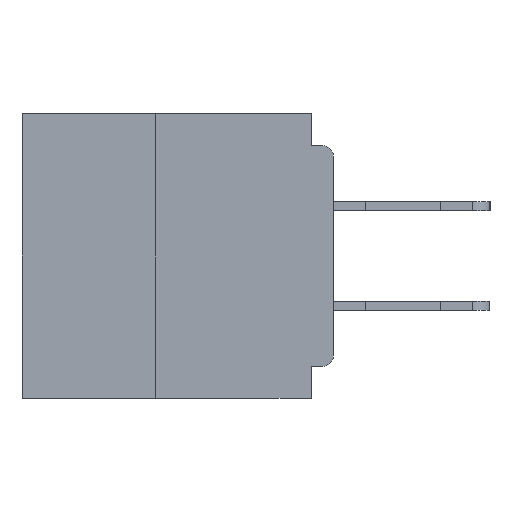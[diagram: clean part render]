
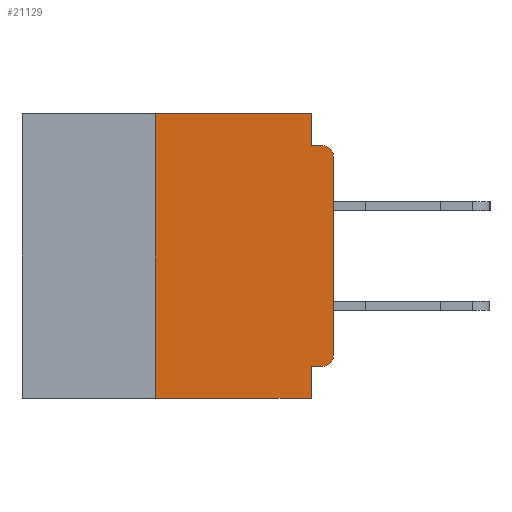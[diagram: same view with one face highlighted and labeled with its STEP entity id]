
A CAD part, left-side view. The second image highlights one B-rep face of the part: STEP entity #21129.
In plain terms, the highlighted planar face has unit normal (-1, 0, 0).
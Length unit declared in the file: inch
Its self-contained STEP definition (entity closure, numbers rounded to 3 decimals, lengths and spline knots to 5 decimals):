
#34 = FACE_OUTER_BOUND ( 'NONE', #45050, .T. ) ;
#398 = CARTESIAN_POINT ( 'NONE',  ( 0., 0.437, -0.4 ) ) ;
#819 = VERTEX_POINT ( 'NONE', #7187 ) ;
#1262 = ORIENTED_EDGE ( 'NONE', *, *, #8777, .F. ) ;
#2060 = LINE ( 'NONE', #12299, #20236 ) ;
#2630 = CARTESIAN_POINT ( 'NONE',  ( 0., 0., 0. ) ) ;
#4308 = VECTOR ( 'NONE', #33841, 39.37008 ) ;
#4326 = LINE ( 'NONE', #37947, #33283 ) ;
#5085 = CARTESIAN_POINT ( 'NONE',  ( 0., 0.031, -0.355 ) ) ;
#5507 = AXIS2_PLACEMENT_3D ( 'NONE', #33290, #11552, #36946 ) ;
#7187 = CARTESIAN_POINT ( 'NONE',  ( 0., 0., -0.34 ) ) ;
#7574 = VERTEX_POINT ( 'NONE', #23682 ) ;
#7761 = DIRECTION ( 'NONE',  ( 0., -1., 0. ) ) ;
#7824 = CARTESIAN_POINT ( 'NONE',  ( 0., 0., -0.045 ) ) ;
#8777 = EDGE_CURVE ( 'NONE', #12521, #19618, #2060, .T. ) ;
#9501 = CARTESIAN_POINT ( 'NONE',  ( 0., 0.437, 0. ) ) ;
#10385 = EDGE_CURVE ( 'NONE', #12523, #819, #18390, .T. ) ;
#10582 = CARTESIAN_POINT ( 'NONE',  ( 0., 0.25, -0.4 ) ) ;
#10930 = CARTESIAN_POINT ( 'NONE',  ( 0., 0., -0.355 ) ) ;
#11438 = DIRECTION ( 'NONE',  ( 0., -1., 0. ) ) ;
#11552 = DIRECTION ( 'NONE',  ( -1., 0., 0. ) ) ;
#11777 = CIRCLE ( 'NONE', #5507, 0.015 ) ;
#12271 = VECTOR ( 'NONE', #7761, 39.37008 ) ;
#12299 = CARTESIAN_POINT ( 'NONE',  ( 0., 0.031, -0.4 ) ) ;
#12521 = VERTEX_POINT ( 'NONE', #5085 ) ;
#12523 = VERTEX_POINT ( 'NONE', #37447 ) ;
#12572 = DIRECTION ( 'NONE',  ( 0., 0., 1. ) ) ;
#13108 = DIRECTION ( 'NONE',  ( 1., 0., 0. ) ) ;
#13409 = ORIENTED_EDGE ( 'NONE', *, *, #14032, .T. ) ;
#13420 = DIRECTION ( 'NONE',  ( 0., 0., 1. ) ) ;
#13845 = VECTOR ( 'NONE', #13420, 39.37008 ) ;
#14032 = EDGE_CURVE ( 'NONE', #819, #38822, #42733, .T. ) ;
#15347 = DIRECTION ( 'NONE',  ( 0., -1., 0. ) ) ;
#15557 = VECTOR ( 'NONE', #32649, 39.37008 ) ;
#15953 = DIRECTION ( 'NONE',  ( 0., 0., -1. ) ) ;
#17094 = VERTEX_POINT ( 'NONE', #43272 ) ;
#17289 = ORIENTED_EDGE ( 'NONE', *, *, #41029, .F. ) ;
#17825 = LINE ( 'NONE', #10930, #15557 ) ;
#18379 = CARTESIAN_POINT ( 'NONE',  ( 0., 0.015, -0.34 ) ) ;
#18390 = CIRCLE ( 'NONE', #34389, 0.015 ) ;
#18498 = EDGE_CURVE ( 'NONE', #33064, #19618, #31568, .T. ) ;
#18512 = ORIENTED_EDGE ( 'NONE', *, *, #38556, .F. ) ;
#18853 = CARTESIAN_POINT ( 'NONE',  ( 0., 0.031, -0.4 ) ) ;
#19017 = AXIS2_PLACEMENT_3D ( 'NONE', #9501, #13108, #38478 ) ;
#19618 = VERTEX_POINT ( 'NONE', #18853 ) ;
#20236 = VECTOR ( 'NONE', #15953, 39.37008 ) ;
#20439 = ORIENTED_EDGE ( 'NONE', *, *, #29828, .T. ) ;
#20630 = VERTEX_POINT ( 'NONE', #31873 ) ;
#20802 = ORIENTED_EDGE ( 'NONE', *, *, #10385, .T. ) ;
#21129 = ADVANCED_FACE ( 'NONE', ( #34 ), #34847, .F. ) ;
#21995 = DIRECTION ( 'NONE',  ( 0., 0., -1. ) ) ;
#22591 = ORIENTED_EDGE ( 'NONE', *, *, #18498, .T. ) ;
#23682 = CARTESIAN_POINT ( 'NONE',  ( 0., 0.031, 0. ) ) ;
#26451 = ORIENTED_EDGE ( 'NONE', *, *, #44359, .F. ) ;
#27883 = VECTOR ( 'NONE', #11438, 39.37008 ) ;
#27938 = CARTESIAN_POINT ( 'NONE',  ( 0., 0., -0.06 ) ) ;
#28305 = CARTESIAN_POINT ( 'NONE',  ( 0., 0.031, -0.045 ) ) ;
#28444 = VERTEX_POINT ( 'NONE', #28305 ) ;
#29364 = ORIENTED_EDGE ( 'NONE', *, *, #30622, .F. ) ;
#29828 = EDGE_CURVE ( 'NONE', #38822, #20630, #11777, .T. ) ;
#30622 = EDGE_CURVE ( 'NONE', #33064, #17094, #4326, .T. ) ;
#31568 = LINE ( 'NONE', #398, #12271 ) ;
#31873 = CARTESIAN_POINT ( 'NONE',  ( 0., 0.015, -0.045 ) ) ;
#32104 = LINE ( 'NONE', #44551, #4308 ) ;
#32649 = DIRECTION ( 'NONE',  ( 0., 1., 0. ) ) ;
#33064 = VERTEX_POINT ( 'NONE', #10582 ) ;
#33283 = VECTOR ( 'NONE', #12572, 39.37008 ) ;
#33290 = CARTESIAN_POINT ( 'NONE',  ( 0., 0.015, -0.06 ) ) ;
#33659 = EDGE_CURVE ( 'NONE', #17094, #7574, #36073, .T. ) ;
#33841 = DIRECTION ( 'NONE',  ( 0., 0., -1. ) ) ;
#34389 = AXIS2_PLACEMENT_3D ( 'NONE', #18379, #43662, #21995 ) ;
#34847 = PLANE ( 'NONE',  #19017 ) ;
#36073 = LINE ( 'NONE', #44314, #43365 ) ;
#36946 = DIRECTION ( 'NONE',  ( 0., 0., -1. ) ) ;
#37035 = ORIENTED_EDGE ( 'NONE', *, *, #33659, .F. ) ;
#37447 = CARTESIAN_POINT ( 'NONE',  ( 0., 0.015, -0.355 ) ) ;
#37554 = LINE ( 'NONE', #7824, #27883 ) ;
#37947 = CARTESIAN_POINT ( 'NONE',  ( 0., 0.25, -0.4 ) ) ;
#38478 = DIRECTION ( 'NONE',  ( 0., 0., -1. ) ) ;
#38556 = EDGE_CURVE ( 'NONE', #7574, #28444, #32104, .T. ) ;
#38822 = VERTEX_POINT ( 'NONE', #27938 ) ;
#41029 = EDGE_CURVE ( 'NONE', #28444, #20630, #37554, .T. ) ;
#42733 = LINE ( 'NONE', #2630, #13845 ) ;
#43272 = CARTESIAN_POINT ( 'NONE',  ( 0., 0.25, 0. ) ) ;
#43365 = VECTOR ( 'NONE', #15347, 39.37008 ) ;
#43662 = DIRECTION ( 'NONE',  ( -1., 0., 0. ) ) ;
#44314 = CARTESIAN_POINT ( 'NONE',  ( 0., 0.437, 0. ) ) ;
#44359 = EDGE_CURVE ( 'NONE', #12523, #12521, #17825, .T. ) ;
#44551 = CARTESIAN_POINT ( 'NONE',  ( 0., 0.031, 0. ) ) ;
#45050 = EDGE_LOOP ( 'NONE', ( #13409, #20439, #17289, #18512, #37035, #29364, #22591, #1262, #26451, #20802 ) ) ;
